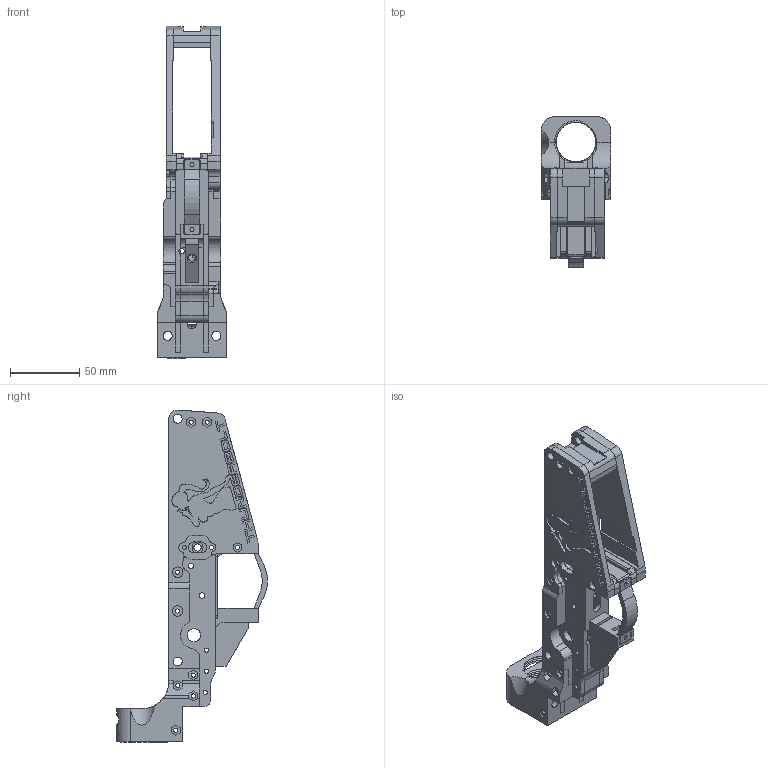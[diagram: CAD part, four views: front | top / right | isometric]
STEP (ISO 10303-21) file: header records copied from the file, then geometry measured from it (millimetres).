
FILE_DESCRIPTION (( 'STEP AP214' ), '1' );
FILE_NAME ('Thunderbolt Assembly.STEP', '2021-08-08T22:48:02', ( '' ), ( '' ), 'SwSTEP 2.0', 'SolidWorks 2020', '' );
FILE_SCHEMA (( 'AUTOMOTIVE_DESIGN' ));
Length unit declared in the file: millimetre
Products named in the file (13): Firebolt_308_Side_Right_Straight; Firebolt_308_Buffer Tower_Split_Arm_Left; Firebolt_308_Mag_Well_Front_Straight; Firebolt_308_Trigger_Guard; Firebolt_308_Mag_Well_Left_Straight_Spooky; Firebolt_308_Buffer Tower_Split_Arm_Right; Firebolt_308_Grip_Part_Straight; Firebolt_308_Mag_Well_Right_Straight; Firebolt_308_Mag_Well_Rear_Straight; Firebolt_308_Fire_Control_Well_Bottom; Thunderbolt Assembly; Firebolt_308_Buffer Tower_Split_Tower; Firebolt_308_Side_Left_Straight
Assembly tree (12 placements, depth 2):
  Thunderbolt Assembly
    Firebolt_308_Trigger_Guard
    Firebolt_308_Fire_Control_Well_Bottom
    Firebolt_308_Mag_Well_Rear_Straight
    Firebolt_308_Mag_Well_Left_Straight_Spooky
    Firebolt_308_Mag_Well_Front_Straight
    Firebolt_308_Mag_Well_Right_Straight
    Firebolt_308_Side_Right_Straight
    Firebolt_308_Side_Left_Straight
    Firebolt_308_Grip_Part_Straight
    Firebolt_308_Buffer Tower_Split_Tower
    Firebolt_308_Buffer Tower_Split_Arm_Left
    Firebolt_308_Buffer Tower_Split_Arm_Right
Bounding box: 50 x 108.63 x 239.08 mm (x, y, z)
Volume: 205364 mm3; surface area: 108886.8 mm2
Topology: 12 solids, 12 shells, 1324 faces, 3648 edges, 2419 vertices
Faces by surface type: plane 666, cylinder 441, bspline 209, cone 8
Entity records: 72922 total; most frequent: CARTESIAN_POINT 39421, ORIENTED_EDGE 7292, DIRECTION 6088, EDGE_CURVE 3646, VERTEX_POINT 2419, LINE 2230, VECTOR 2230, AXIS2_PLACEMENT_3D 1929
